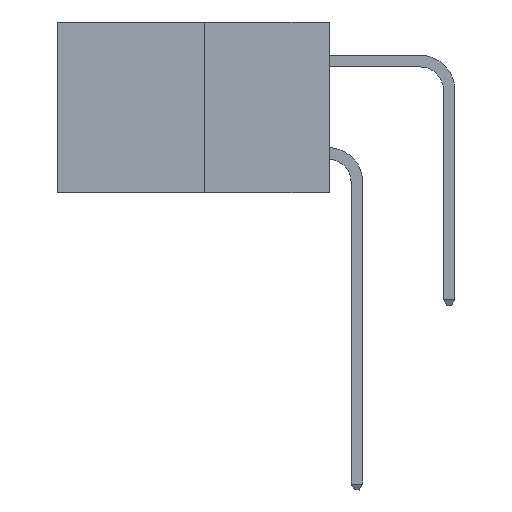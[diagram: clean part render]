
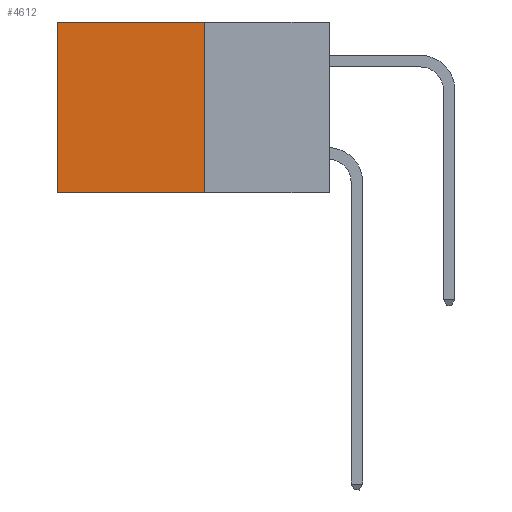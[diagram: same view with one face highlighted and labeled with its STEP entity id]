
A CAD part, left-side view. The second image highlights one B-rep face of the part: STEP entity #4612.
In plain terms, the highlighted planar face has unit normal (-1, 0, 0).
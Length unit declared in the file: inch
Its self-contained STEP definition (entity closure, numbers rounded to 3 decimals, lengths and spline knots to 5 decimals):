
#108 = DIRECTION ( 'NONE',  ( 0., 1., 0. ) ) ;
#393 = DIRECTION ( 'NONE',  ( 0., 0., -1. ) ) ;
#979 = LINE ( 'NONE', #1185, #3680 ) ;
#1185 = CARTESIAN_POINT ( 'NONE',  ( 0.277, 0.27, 0. ) ) ;
#1740 = ORIENTED_EDGE ( 'NONE', *, *, #2722, .T. ) ;
#1776 = AXIS2_PLACEMENT_3D ( 'NONE', #5082, #4284, #4135 ) ;
#1834 = ORIENTED_EDGE ( 'NONE', *, *, #3575, .F. ) ;
#1989 = ORIENTED_EDGE ( 'NONE', *, *, #2412, .T. ) ;
#2043 = CARTESIAN_POINT ( 'NONE',  ( 0.277, 0.27, 0. ) ) ;
#2412 = EDGE_CURVE ( 'NONE', #5583, #6587, #979, .T. ) ;
#2547 = VECTOR ( 'NONE', #3895, 39.37008 ) ;
#2722 = EDGE_CURVE ( 'NONE', #6587, #8392, #8976, .T. ) ;
#3575 = EDGE_CURVE ( 'NONE', #4061, #8392, #5884, .T. ) ;
#3612 = FACE_OUTER_BOUND ( 'NONE', #8665, .T. ) ;
#3680 = VECTOR ( 'NONE', #108, 39.37008 ) ;
#3710 = ORIENTED_EDGE ( 'NONE', *, *, #4442, .F. ) ;
#3895 = DIRECTION ( 'NONE',  ( 0., 1., 0. ) ) ;
#4061 = VERTEX_POINT ( 'NONE', #9517 ) ;
#4135 = DIRECTION ( 'NONE',  ( 0., 0., -1. ) ) ;
#4284 = DIRECTION ( 'NONE',  ( 1., 0., 0. ) ) ;
#4442 = EDGE_CURVE ( 'NONE', #5583, #4061, #4849, .T. ) ;
#4543 = CARTESIAN_POINT ( 'NONE',  ( 0.277, 0.59, 0. ) ) ;
#4612 = ADVANCED_FACE ( 'NONE', ( #3612 ), #4812, .F. ) ;
#4812 = PLANE ( 'NONE',  #1776 ) ;
#4849 = LINE ( 'NONE', #6029, #8249 ) ;
#5082 = CARTESIAN_POINT ( 'NONE',  ( 0.277, 0.27, -0.37 ) ) ;
#5120 = CARTESIAN_POINT ( 'NONE',  ( 0.277, 0.27, -0.37 ) ) ;
#5583 = VERTEX_POINT ( 'NONE', #2043 ) ;
#5884 = LINE ( 'NONE', #5120, #2547 ) ;
#6029 = CARTESIAN_POINT ( 'NONE',  ( 0.277, 0.27, -0.37 ) ) ;
#6587 = VERTEX_POINT ( 'NONE', #4543 ) ;
#7324 = VECTOR ( 'NONE', #9383, 39.37008 ) ;
#8249 = VECTOR ( 'NONE', #393, 39.37008 ) ;
#8392 = VERTEX_POINT ( 'NONE', #9065 ) ;
#8665 = EDGE_LOOP ( 'NONE', ( #1740, #1834, #3710, #1989 ) ) ;
#8976 = LINE ( 'NONE', #9405, #7324 ) ;
#9065 = CARTESIAN_POINT ( 'NONE',  ( 0.277, 0.59, -0.37 ) ) ;
#9383 = DIRECTION ( 'NONE',  ( 0., 0., -1. ) ) ;
#9405 = CARTESIAN_POINT ( 'NONE',  ( 0.277, 0.59, -0.37 ) ) ;
#9517 = CARTESIAN_POINT ( 'NONE',  ( 0.277, 0.27, -0.37 ) ) ;
